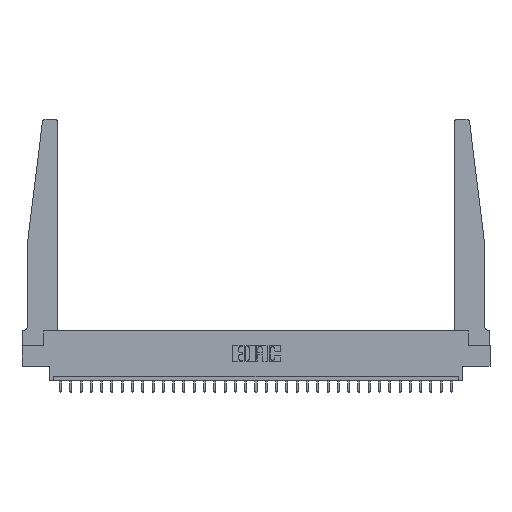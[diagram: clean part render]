
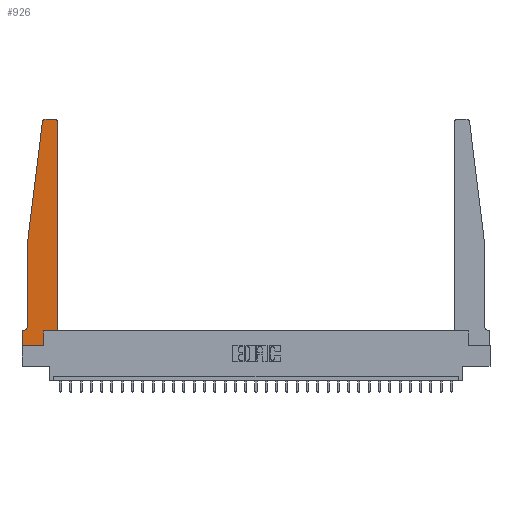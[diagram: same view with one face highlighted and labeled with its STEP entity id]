
A CAD part, top view. The second image highlights one B-rep face of the part: STEP entity #926.
In plain terms, the highlighted planar face has unit normal (0, 0, 1).
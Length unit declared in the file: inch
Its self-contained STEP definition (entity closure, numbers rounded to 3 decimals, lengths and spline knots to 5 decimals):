
#21 = EDGE_CURVE ( 'NONE', #17000, #28381, #5123, .T. ) ;
#22 = CARTESIAN_POINT ( 'NONE',  ( 0.2605, 0., 0.37 ) ) ;
#35 = ORIENTED_EDGE ( 'NONE', *, *, #6065, .T. ) ;
#117 = CARTESIAN_POINT ( 'NONE',  ( 0.2605, 0.18, 0.37 ) ) ;
#263 = CARTESIAN_POINT ( 'NONE',  ( 0.27653, 2.72, 0.37 ) ) ;
#280 = CARTESIAN_POINT ( 'NONE',  ( 0.2605, 0.18, 0.37 ) ) ;
#805 = EDGE_CURVE ( 'NONE', #26974, #17274, #27794, .T. ) ;
#926 = ADVANCED_FACE ( 'NONE', ( #11461 ), #10516, .T. ) ;
#2907 = DIRECTION ( 'NONE',  ( 0., 0., 1. ) ) ;
#3447 = VERTEX_POINT ( 'NONE', #9511 ) ;
#3492 = CARTESIAN_POINT ( 'NONE',  ( 0., 0.1875, 0.37 ) ) ;
#3799 = DIRECTION ( 'NONE',  ( -1., 0., 0. ) ) ;
#3818 = ORIENTED_EDGE ( 'NONE', *, *, #14417, .T. ) ;
#3949 = CARTESIAN_POINT ( 'NONE',  ( 0.015, 0.2375, 0.37 ) ) ;
#3993 = ORIENTED_EDGE ( 'NONE', *, *, #21, .T. ) ;
#4163 = CARTESIAN_POINT ( 'NONE',  ( 0., 0., 0.37 ) ) ;
#4313 = LINE ( 'NONE', #4163, #21703 ) ;
#4840 = CARTESIAN_POINT ( 'NONE',  ( 0.395, 2.72, 0.37 ) ) ;
#5059 = CARTESIAN_POINT ( 'NONE',  ( 0.425, 0.18, 0.37 ) ) ;
#5123 = CIRCLE ( 'NONE', #15772, 0.05 ) ;
#5221 = LINE ( 'NONE', #11778, #29109 ) ;
#5557 = EDGE_LOOP ( 'NONE', ( #10886, #10944, #17381, #29890, #3993, #35, #13530, #11683, #9819, #27347, #7254, #3818 ) ) ;
#5615 = VECTOR ( 'NONE', #20675, 39.37008 ) ;
#5718 = EDGE_CURVE ( 'NONE', #3447, #18141, #18176, .T. ) ;
#5829 = EDGE_CURVE ( 'NONE', #9098, #27414, #11832, .T. ) ;
#6065 = EDGE_CURVE ( 'NONE', #28381, #3447, #12128, .T. ) ;
#6124 = EDGE_CURVE ( 'NONE', #26843, #17000, #10600, .T. ) ;
#6266 = CARTESIAN_POINT ( 'NONE',  ( 0.065, 0.2375, 0.37 ) ) ;
#6467 = DIRECTION ( 'NONE',  ( 0., -1., 0. ) ) ;
#6646 = CARTESIAN_POINT ( 'NONE',  ( 0., 0., 0.37 ) ) ;
#6886 = LINE ( 'NONE', #5059, #16229 ) ;
#7248 = CARTESIAN_POINT ( 'NONE',  ( 0.425, 2.72, 0.37 ) ) ;
#7254 = ORIENTED_EDGE ( 'NONE', *, *, #24931, .T. ) ;
#7323 = CARTESIAN_POINT ( 'NONE',  ( 0.015, 0.1875, 0.37 ) ) ;
#7358 = DIRECTION ( 'NONE',  ( 1., 0., 0. ) ) ;
#7703 = DIRECTION ( 'NONE',  ( -1., 0., 0. ) ) ;
#8640 = VERTEX_POINT ( 'NONE', #18131 ) ;
#9098 = VERTEX_POINT ( 'NONE', #22 ) ;
#9107 = DIRECTION ( 'NONE',  ( 0., 1., 0. ) ) ;
#9416 = DIRECTION ( 'NONE',  ( 1., 0., 0. ) ) ;
#9511 = CARTESIAN_POINT ( 'NONE',  ( 0., 0.1875, 0.37 ) ) ;
#9819 = ORIENTED_EDGE ( 'NONE', *, *, #5829, .T. ) ;
#9930 = DIRECTION ( 'NONE',  ( 1., 0., 0. ) ) ;
#10202 = CARTESIAN_POINT ( 'NONE',  ( 0.27653, 2.75, 0.37 ) ) ;
#10516 = PLANE ( 'NONE',  #16782 ) ;
#10600 = LINE ( 'NONE', #29205, #19608 ) ;
#10695 = CARTESIAN_POINT ( 'NONE',  ( 0., 0., 0.37 ) ) ;
#10886 = ORIENTED_EDGE ( 'NONE', *, *, #805, .T. ) ;
#10944 = ORIENTED_EDGE ( 'NONE', *, *, #18775, .T. ) ;
#11025 = DIRECTION ( 'NONE',  ( 1., 0., 0. ) ) ;
#11103 = EDGE_CURVE ( 'NONE', #18141, #9098, #4313, .T. ) ;
#11461 = FACE_OUTER_BOUND ( 'NONE', #5557, .T. ) ;
#11683 = ORIENTED_EDGE ( 'NONE', *, *, #11103, .T. ) ;
#11778 = CARTESIAN_POINT ( 'NONE',  ( 0.425, 0.18, 0.37 ) ) ;
#11832 = LINE ( 'NONE', #280, #18146 ) ;
#11852 = CARTESIAN_POINT ( 'NONE',  ( 0.395, 2.75, 0.37 ) ) ;
#12027 = AXIS2_PLACEMENT_3D ( 'NONE', #4840, #20915, #9416 ) ;
#12128 = LINE ( 'NONE', #14832, #19100 ) ;
#13524 = DIRECTION ( 'NONE',  ( 0., 0., -1. ) ) ;
#13530 = ORIENTED_EDGE ( 'NONE', *, *, #5718, .T. ) ;
#14057 = VERTEX_POINT ( 'NONE', #19491 ) ;
#14417 = EDGE_CURVE ( 'NONE', #16220, #26974, #19238, .T. ) ;
#14595 = AXIS2_PLACEMENT_3D ( 'NONE', #263, #15740, #24974 ) ;
#14832 = CARTESIAN_POINT ( 'NONE',  ( 0.065, 0.1875, 0.37 ) ) ;
#15740 = DIRECTION ( 'NONE',  ( 0., 0., 1. ) ) ;
#15772 = AXIS2_PLACEMENT_3D ( 'NONE', #3949, #13524, #3799 ) ;
#15896 = LINE ( 'NONE', #27714, #16078 ) ;
#15986 = DIRECTION ( 'NONE',  ( 0., 1., 0. ) ) ;
#16078 = VECTOR ( 'NONE', #20742, 39.37008 ) ;
#16220 = VERTEX_POINT ( 'NONE', #7248 ) ;
#16229 = VECTOR ( 'NONE', #15986, 39.37008 ) ;
#16782 = AXIS2_PLACEMENT_3D ( 'NONE', #3492, #2907, #9930 ) ;
#17000 = VERTEX_POINT ( 'NONE', #6266 ) ;
#17274 = VERTEX_POINT ( 'NONE', #10202 ) ;
#17381 = ORIENTED_EDGE ( 'NONE', *, *, #27423, .T. ) ;
#18131 = CARTESIAN_POINT ( 'NONE',  ( 0.425, 0.18, 0.37 ) ) ;
#18141 = VERTEX_POINT ( 'NONE', #10695 ) ;
#18146 = VECTOR ( 'NONE', #9107, 39.37008 ) ;
#18176 = LINE ( 'NONE', #6646, #26374 ) ;
#18775 = EDGE_CURVE ( 'NONE', #17274, #14057, #20887, .T. ) ;
#19100 = VECTOR ( 'NONE', #7703, 39.37008 ) ;
#19238 = CIRCLE ( 'NONE', #12027, 0.03 ) ;
#19491 = CARTESIAN_POINT ( 'NONE',  ( 0.24675, 2.72367, 0.37 ) ) ;
#19608 = VECTOR ( 'NONE', #6467, 39.37008 ) ;
#19849 = DIRECTION ( 'NONE',  ( 0., -1., 0. ) ) ;
#20675 = DIRECTION ( 'NONE',  ( -1., 0., 0. ) ) ;
#20742 = DIRECTION ( 'NONE',  ( -0.122, -0.992, 0. ) ) ;
#20821 = CARTESIAN_POINT ( 'NONE',  ( 0.25, 2.75, 0.37 ) ) ;
#20887 = CIRCLE ( 'NONE', #14595, 0.03 ) ;
#20915 = DIRECTION ( 'NONE',  ( 0., 0., 1. ) ) ;
#21703 = VECTOR ( 'NONE', #11025, 39.37008 ) ;
#24931 = EDGE_CURVE ( 'NONE', #8640, #16220, #6886, .T. ) ;
#24974 = DIRECTION ( 'NONE',  ( 1., 0., 0. ) ) ;
#26374 = VECTOR ( 'NONE', #19849, 39.37008 ) ;
#26724 = EDGE_CURVE ( 'NONE', #27414, #8640, #5221, .T. ) ;
#26843 = VERTEX_POINT ( 'NONE', #29148 ) ;
#26974 = VERTEX_POINT ( 'NONE', #11852 ) ;
#27347 = ORIENTED_EDGE ( 'NONE', *, *, #26724, .T. ) ;
#27414 = VERTEX_POINT ( 'NONE', #117 ) ;
#27423 = EDGE_CURVE ( 'NONE', #14057, #26843, #15896, .T. ) ;
#27714 = CARTESIAN_POINT ( 'NONE',  ( 0.065, 1.25, 0.37 ) ) ;
#27794 = LINE ( 'NONE', #20821, #5615 ) ;
#28381 = VERTEX_POINT ( 'NONE', #7323 ) ;
#29109 = VECTOR ( 'NONE', #7358, 39.37008 ) ;
#29148 = CARTESIAN_POINT ( 'NONE',  ( 0.065, 1.25, 0.37 ) ) ;
#29205 = CARTESIAN_POINT ( 'NONE',  ( 0.065, 1.25, 0.37 ) ) ;
#29890 = ORIENTED_EDGE ( 'NONE', *, *, #6124, .T. ) ;
